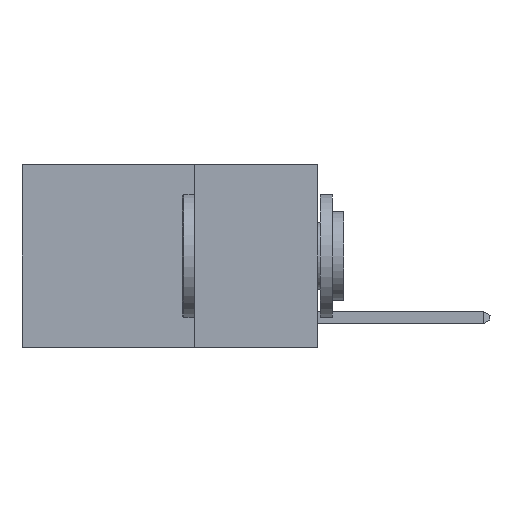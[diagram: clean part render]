
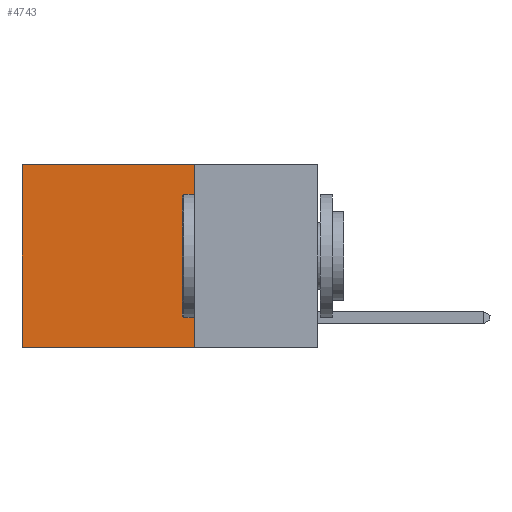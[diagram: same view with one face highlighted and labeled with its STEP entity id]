
A CAD part, left-side view. The second image highlights one B-rep face of the part: STEP entity #4743.
In plain terms, the highlighted planar face has unit normal (-1, 0, 0).
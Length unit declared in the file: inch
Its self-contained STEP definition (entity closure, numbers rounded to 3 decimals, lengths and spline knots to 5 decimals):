
#230 = VECTOR ( 'NONE', #320, 39.37008 ) ;
#320 = DIRECTION ( 'NONE',  ( 0., 0., -1. ) ) ;
#350 = ORIENTED_EDGE ( 'NONE', *, *, #12130, .F. ) ;
#964 = CARTESIAN_POINT ( 'NONE',  ( 0.2625, 0.25, 0. ) ) ;
#2907 = CARTESIAN_POINT ( 'NONE',  ( 0.2625, 0.6, 0. ) ) ;
#2975 = VERTEX_POINT ( 'NONE', #2907 ) ;
#4071 = EDGE_LOOP ( 'NONE', ( #12183, #12969, #350, #10500 ) ) ;
#4240 = LINE ( 'NONE', #8295, #230 ) ;
#4628 = VECTOR ( 'NONE', #14006, 39.37008 ) ;
#4743 = ADVANCED_FACE ( 'NONE', ( #6094 ), #12710, .F. ) ;
#4760 = EDGE_CURVE ( 'NONE', #2975, #15093, #11165, .T. ) ;
#6094 = FACE_OUTER_BOUND ( 'NONE', #4071, .T. ) ;
#6594 = CARTESIAN_POINT ( 'NONE',  ( 0.2625, 0.6, -0.37 ) ) ;
#6710 = DIRECTION ( 'NONE',  ( 0., 1., 0. ) ) ;
#8295 = CARTESIAN_POINT ( 'NONE',  ( 0.2625, 0.25, 0. ) ) ;
#8736 = CARTESIAN_POINT ( 'NONE',  ( 0.2625, 0.25, -0.37 ) ) ;
#8985 = EDGE_CURVE ( 'NONE', #16632, #15093, #11628, .T. ) ;
#9133 = VERTEX_POINT ( 'NONE', #14991 ) ;
#9560 = CARTESIAN_POINT ( 'NONE',  ( 0.2625, 0.25, -0.37 ) ) ;
#9682 = LINE ( 'NONE', #12513, #10657 ) ;
#10148 = VECTOR ( 'NONE', #6710, 39.37008 ) ;
#10219 = CARTESIAN_POINT ( 'NONE',  ( 0.2625, 0.6, 0. ) ) ;
#10500 = ORIENTED_EDGE ( 'NONE', *, *, #15232, .T. ) ;
#10657 = VECTOR ( 'NONE', #12265, 39.37008 ) ;
#11165 = LINE ( 'NONE', #10219, #4628 ) ;
#11331 = DIRECTION ( 'NONE',  ( 1., 0., 0. ) ) ;
#11628 = LINE ( 'NONE', #9560, #10148 ) ;
#12130 = EDGE_CURVE ( 'NONE', #9133, #16632, #4240, .T. ) ;
#12183 = ORIENTED_EDGE ( 'NONE', *, *, #4760, .T. ) ;
#12265 = DIRECTION ( 'NONE',  ( 0., 1., 0. ) ) ;
#12513 = CARTESIAN_POINT ( 'NONE',  ( 0.2625, 0.25, 0. ) ) ;
#12710 = PLANE ( 'NONE',  #13129 ) ;
#12969 = ORIENTED_EDGE ( 'NONE', *, *, #8985, .F. ) ;
#13129 = AXIS2_PLACEMENT_3D ( 'NONE', #964, #11331, #14168 ) ;
#14006 = DIRECTION ( 'NONE',  ( 0., 0., -1. ) ) ;
#14168 = DIRECTION ( 'NONE',  ( 0., 0., -1. ) ) ;
#14991 = CARTESIAN_POINT ( 'NONE',  ( 0.2625, 0.25, 0. ) ) ;
#15093 = VERTEX_POINT ( 'NONE', #6594 ) ;
#15232 = EDGE_CURVE ( 'NONE', #9133, #2975, #9682, .T. ) ;
#16632 = VERTEX_POINT ( 'NONE', #8736 ) ;
